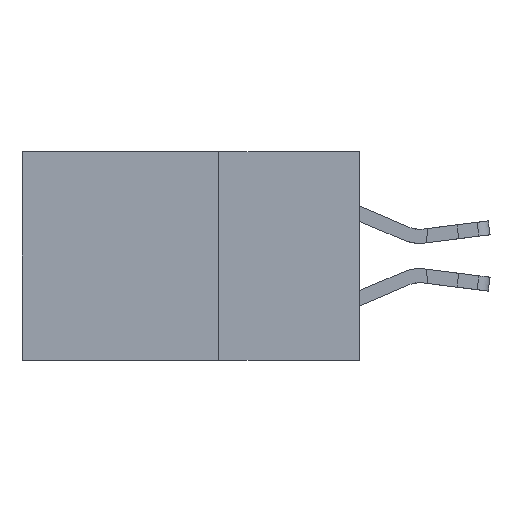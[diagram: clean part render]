
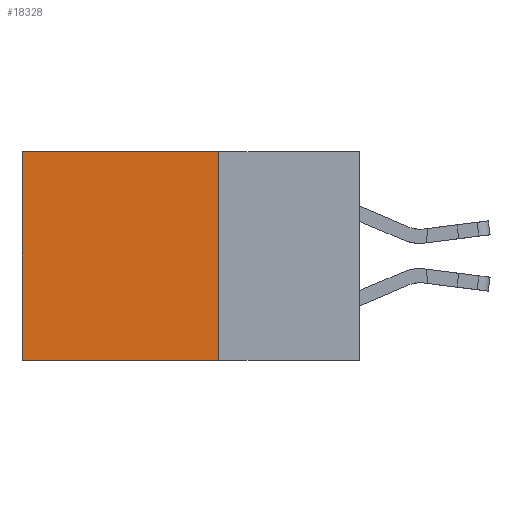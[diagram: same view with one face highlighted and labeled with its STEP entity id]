
A CAD part, left-side view. The second image highlights one B-rep face of the part: STEP entity #18328.
In plain terms, the highlighted planar face has unit normal (-1, 0, 0).
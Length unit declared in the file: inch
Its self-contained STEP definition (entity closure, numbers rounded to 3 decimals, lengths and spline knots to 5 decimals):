
#243 = EDGE_CURVE ( 'NONE', #16416, #24011, #6762, .T. ) ;
#270 = LINE ( 'NONE', #18053, #13868 ) ;
#729 = EDGE_CURVE ( 'NONE', #23985, #16785, #270, .T. ) ;
#1827 = EDGE_LOOP ( 'NONE', ( #12340, #6529, #10140, #22275 ) ) ;
#5453 = CARTESIAN_POINT ( 'NONE',  ( 0.2875, 0.6, 0. ) ) ;
#6529 = ORIENTED_EDGE ( 'NONE', *, *, #729, .F. ) ;
#6762 = LINE ( 'NONE', #14952, #30934 ) ;
#6960 = VECTOR ( 'NONE', #13400, 39.37008 ) ;
#7672 = LINE ( 'NONE', #27910, #6960 ) ;
#7814 = CARTESIAN_POINT ( 'NONE',  ( 0.2875, 0.25, 0. ) ) ;
#9768 = VECTOR ( 'NONE', #29577, 39.37008 ) ;
#10140 = ORIENTED_EDGE ( 'NONE', *, *, #13935, .F. ) ;
#12340 = ORIENTED_EDGE ( 'NONE', *, *, #24195, .T. ) ;
#13400 = DIRECTION ( 'NONE',  ( 0., 0., -1. ) ) ;
#13868 = VECTOR ( 'NONE', #17831, 39.37008 ) ;
#13935 = EDGE_CURVE ( 'NONE', #16416, #23985, #16161, .T. ) ;
#14952 = CARTESIAN_POINT ( 'NONE',  ( 0.2875, 0.25, 0. ) ) ;
#16161 = LINE ( 'NONE', #7814, #9768 ) ;
#16416 = VERTEX_POINT ( 'NONE', #28448 ) ;
#16785 = VERTEX_POINT ( 'NONE', #28370 ) ;
#17831 = DIRECTION ( 'NONE',  ( 0., 1., 0. ) ) ;
#18053 = CARTESIAN_POINT ( 'NONE',  ( 0.2875, 0.25, -0.37 ) ) ;
#18328 = ADVANCED_FACE ( 'NONE', ( #22922 ), #19082, .F. ) ;
#18436 = DIRECTION ( 'NONE',  ( 0., 0., -1. ) ) ;
#18772 = DIRECTION ( 'NONE',  ( 1., 0., 0. ) ) ;
#19082 = PLANE ( 'NONE',  #29401 ) ;
#22275 = ORIENTED_EDGE ( 'NONE', *, *, #243, .T. ) ;
#22452 = CARTESIAN_POINT ( 'NONE',  ( 0.2875, 0.25, -0.37 ) ) ;
#22922 = FACE_OUTER_BOUND ( 'NONE', #1827, .T. ) ;
#23985 = VERTEX_POINT ( 'NONE', #22452 ) ;
#24011 = VERTEX_POINT ( 'NONE', #5453 ) ;
#24195 = EDGE_CURVE ( 'NONE', #24011, #16785, #7672, .T. ) ;
#24505 = DIRECTION ( 'NONE',  ( 0., 1., 0. ) ) ;
#27910 = CARTESIAN_POINT ( 'NONE',  ( 0.2875, 0.6, 0. ) ) ;
#28370 = CARTESIAN_POINT ( 'NONE',  ( 0.2875, 0.6, -0.37 ) ) ;
#28448 = CARTESIAN_POINT ( 'NONE',  ( 0.2875, 0.25, 0. ) ) ;
#29401 = AXIS2_PLACEMENT_3D ( 'NONE', #31201, #18772, #18436 ) ;
#29577 = DIRECTION ( 'NONE',  ( 0., 0., -1. ) ) ;
#30934 = VECTOR ( 'NONE', #24505, 39.37008 ) ;
#31201 = CARTESIAN_POINT ( 'NONE',  ( 0.2875, 0.25, 0. ) ) ;
